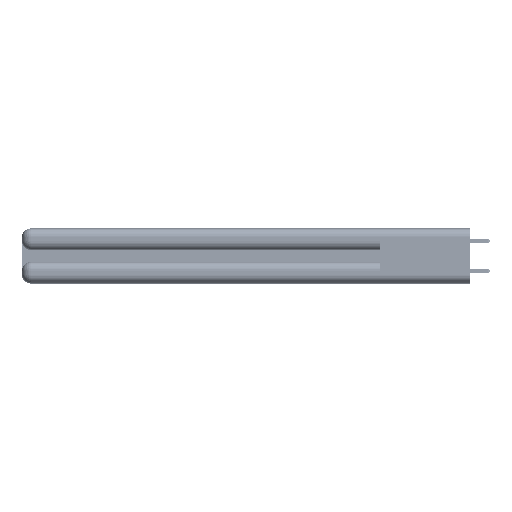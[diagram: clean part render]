
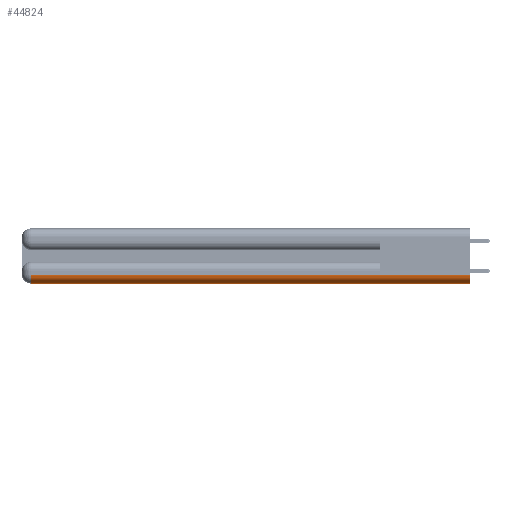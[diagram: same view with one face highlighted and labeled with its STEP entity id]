
A CAD part, left-side view. The second image highlights one B-rep face of the part: STEP entity #44824.
In plain terms, the highlighted cylindrical face has radius 1.524 mm (diameter 3.048 mm), a partial arc.
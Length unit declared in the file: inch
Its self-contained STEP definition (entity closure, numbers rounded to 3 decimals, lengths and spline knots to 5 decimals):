
#212 = DIRECTION ( 'NONE',  ( 0., -1., 0. ) ) ;
#2679 = DIRECTION ( 'NONE',  ( 0., 0., 1. ) ) ;
#2834 = EDGE_CURVE ( 'NONE', #35128, #47074, #30782, .T. ) ;
#2994 = DIRECTION ( 'NONE',  ( 0., 1., 0. ) ) ;
#4697 = CARTESIAN_POINT ( 'NONE',  ( 0.06, 2.94, 0.06 ) ) ;
#7042 = VECTOR ( 'NONE', #212, 39.37008 ) ;
#8910 = DIRECTION ( 'NONE',  ( 0., 0., 1. ) ) ;
#9062 = VERTEX_POINT ( 'NONE', #45390 ) ;
#9463 = CIRCLE ( 'NONE', #41159, 0.06 ) ;
#9654 = EDGE_CURVE ( 'NONE', #9062, #35128, #9463, .T. ) ;
#12738 = CARTESIAN_POINT ( 'NONE',  ( 0.06, 0., 0.06 ) ) ;
#16482 = VERTEX_POINT ( 'NONE', #18547 ) ;
#17002 = DIRECTION ( 'NONE',  ( 0., 0., 1. ) ) ;
#18227 = EDGE_LOOP ( 'NONE', ( #52610, #42776, #36910, #49375 ) ) ;
#18547 = CARTESIAN_POINT ( 'NONE',  ( 0.06, 0., 0. ) ) ;
#19763 = CARTESIAN_POINT ( 'NONE',  ( 0.06, 3., 0. ) ) ;
#25890 = VECTOR ( 'NONE', #2994, 39.37008 ) ;
#27512 = EDGE_CURVE ( 'NONE', #16482, #9062, #37088, .T. ) ;
#27898 = DIRECTION ( 'NONE',  ( 0., -1., 0. ) ) ;
#30283 = CARTESIAN_POINT ( 'NONE',  ( 0., 0., 0.06 ) ) ;
#30782 = LINE ( 'NONE', #33906, #7042 ) ;
#33906 = CARTESIAN_POINT ( 'NONE',  ( 0., 0., 0.06 ) ) ;
#34143 = DIRECTION ( 'NONE',  ( 0., 1., 0. ) ) ;
#34757 = CYLINDRICAL_SURFACE ( 'NONE', #49066, 0.06 ) ;
#35128 = VERTEX_POINT ( 'NONE', #40321 ) ;
#35760 = CIRCLE ( 'NONE', #39569, 0.06 ) ;
#36910 = ORIENTED_EDGE ( 'NONE', *, *, #9654, .F. ) ;
#37088 = LINE ( 'NONE', #19763, #25890 ) ;
#39569 = AXIS2_PLACEMENT_3D ( 'NONE', #53026, #27898, #2679 ) ;
#40321 = CARTESIAN_POINT ( 'NONE',  ( 0., 2.94, 0.06 ) ) ;
#41159 = AXIS2_PLACEMENT_3D ( 'NONE', #4697, #34143, #8910 ) ;
#42232 = EDGE_CURVE ( 'NONE', #47074, #16482, #35760, .T. ) ;
#42776 = ORIENTED_EDGE ( 'NONE', *, *, #2834, .F. ) ;
#44824 = ADVANCED_FACE ( 'NONE', ( #48508 ), #34757, .T. ) ;
#45390 = CARTESIAN_POINT ( 'NONE',  ( 0.06, 2.94, 0. ) ) ;
#46348 = DIRECTION ( 'NONE',  ( 0., 1., 0. ) ) ;
#47074 = VERTEX_POINT ( 'NONE', #30283 ) ;
#48508 = FACE_OUTER_BOUND ( 'NONE', #18227, .T. ) ;
#49066 = AXIS2_PLACEMENT_3D ( 'NONE', #12738, #46348, #17002 ) ;
#49375 = ORIENTED_EDGE ( 'NONE', *, *, #27512, .F. ) ;
#52610 = ORIENTED_EDGE ( 'NONE', *, *, #42232, .F. ) ;
#53026 = CARTESIAN_POINT ( 'NONE',  ( 0.06, 0., 0.06 ) ) ;
